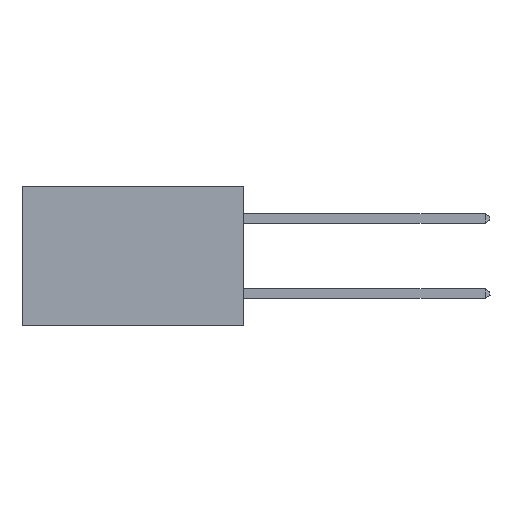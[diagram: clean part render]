
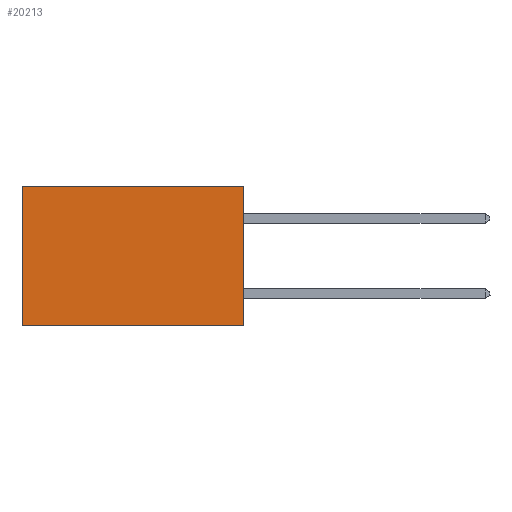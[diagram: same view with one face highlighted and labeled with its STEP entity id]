
A CAD part, left-side view. The second image highlights one B-rep face of the part: STEP entity #20213.
In plain terms, the highlighted planar face has unit normal (-1, 0, 0).
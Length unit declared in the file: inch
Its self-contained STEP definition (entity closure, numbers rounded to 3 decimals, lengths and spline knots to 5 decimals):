
#258 = EDGE_CURVE ( 'NONE', #23551, #12069, #18756, .T. ) ;
#599 = CARTESIAN_POINT ( 'NONE',  ( 0.277, 0., -0.37 ) ) ;
#989 = CARTESIAN_POINT ( 'NONE',  ( 0.277, 0., 0. ) ) ;
#2103 = PLANE ( 'NONE',  #8978 ) ;
#2692 = DIRECTION ( 'NONE',  ( 0., 0., -1. ) ) ;
#3279 = LINE ( 'NONE', #25295, #15334 ) ;
#3627 = VECTOR ( 'NONE', #10953, 39.37008 ) ;
#3942 = ORIENTED_EDGE ( 'NONE', *, *, #11704, .T. ) ;
#4023 = EDGE_LOOP ( 'NONE', ( #3942, #5366, #10710, #8048 ) ) ;
#4095 = CARTESIAN_POINT ( 'NONE',  ( 0.277, 0., 0. ) ) ;
#4381 = DIRECTION ( 'NONE',  ( 0., 0., -1. ) ) ;
#5366 = ORIENTED_EDGE ( 'NONE', *, *, #5530, .F. ) ;
#5530 = EDGE_CURVE ( 'NONE', #12069, #19377, #24508, .T. ) ;
#7892 = CARTESIAN_POINT ( 'NONE',  ( 0.277, 0., -0.37 ) ) ;
#8048 = ORIENTED_EDGE ( 'NONE', *, *, #22241, .T. ) ;
#8835 = DIRECTION ( 'NONE',  ( 0., 1., 0. ) ) ;
#8902 = VERTEX_POINT ( 'NONE', #20594 ) ;
#8978 = AXIS2_PLACEMENT_3D ( 'NONE', #13420, #17914, #4381 ) ;
#10710 = ORIENTED_EDGE ( 'NONE', *, *, #258, .F. ) ;
#10953 = DIRECTION ( 'NONE',  ( 0., 1., 0. ) ) ;
#11704 = EDGE_CURVE ( 'NONE', #8902, #19377, #3279, .T. ) ;
#11871 = DIRECTION ( 'NONE',  ( 0., 0., -1. ) ) ;
#12069 = VERTEX_POINT ( 'NONE', #19794 ) ;
#13420 = CARTESIAN_POINT ( 'NONE',  ( 0.277, 0., -0.37 ) ) ;
#15334 = VECTOR ( 'NONE', #11871, 39.37008 ) ;
#17914 = DIRECTION ( 'NONE',  ( 1., 0., 0. ) ) ;
#18040 = VECTOR ( 'NONE', #2692, 39.37008 ) ;
#18227 = FACE_OUTER_BOUND ( 'NONE', #4023, .T. ) ;
#18531 = VECTOR ( 'NONE', #8835, 39.37008 ) ;
#18756 = LINE ( 'NONE', #599, #18040 ) ;
#19377 = VERTEX_POINT ( 'NONE', #24709 ) ;
#19794 = CARTESIAN_POINT ( 'NONE',  ( 0.277, 0., -0.37 ) ) ;
#20213 = ADVANCED_FACE ( 'NONE', ( #18227 ), #2103, .F. ) ;
#20594 = CARTESIAN_POINT ( 'NONE',  ( 0.277, 0.59, 0. ) ) ;
#22241 = EDGE_CURVE ( 'NONE', #23551, #8902, #28302, .T. ) ;
#23551 = VERTEX_POINT ( 'NONE', #989 ) ;
#24508 = LINE ( 'NONE', #7892, #18531 ) ;
#24709 = CARTESIAN_POINT ( 'NONE',  ( 0.277, 0.59, -0.37 ) ) ;
#25295 = CARTESIAN_POINT ( 'NONE',  ( 0.277, 0.59, -0.37 ) ) ;
#28302 = LINE ( 'NONE', #4095, #3627 ) ;
